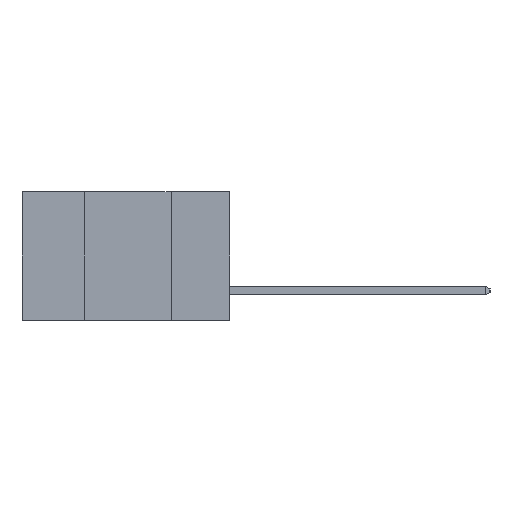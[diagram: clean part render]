
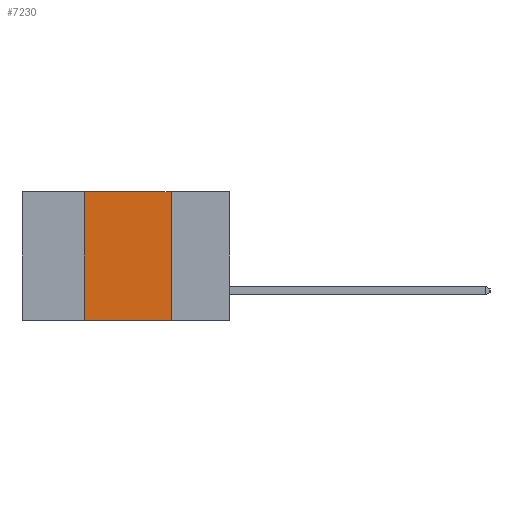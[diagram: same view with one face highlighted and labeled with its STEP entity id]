
A CAD part, left-side view. The second image highlights one B-rep face of the part: STEP entity #7230.
In plain terms, the highlighted planar face has unit normal (-1, 0, 0).
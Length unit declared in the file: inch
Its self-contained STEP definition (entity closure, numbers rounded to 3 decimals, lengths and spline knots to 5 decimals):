
#429 = VECTOR ( 'NONE', #4932, 39.37008 ) ;
#771 = AXIS2_PLACEMENT_3D ( 'NONE', #3577, #3506, #3486 ) ;
#937 = LINE ( 'NONE', #2369, #7788 ) ;
#1126 = FACE_OUTER_BOUND ( 'NONE', #3148, .T. ) ;
#1484 = VECTOR ( 'NONE', #6190, 39.37008 ) ;
#2097 = CARTESIAN_POINT ( 'NONE',  ( 0., 0.17, -0.37 ) ) ;
#2140 = EDGE_CURVE ( 'NONE', #3758, #3508, #8169, .T. ) ;
#2243 = DIRECTION ( 'NONE',  ( 0., -1., 0. ) ) ;
#2342 = LINE ( 'NONE', #4279, #429 ) ;
#2369 = CARTESIAN_POINT ( 'NONE',  ( 0., 0.6, -0.37 ) ) ;
#2577 = VERTEX_POINT ( 'NONE', #4008 ) ;
#3101 = LINE ( 'NONE', #8383, #1484 ) ;
#3103 = VECTOR ( 'NONE', #4259, 39.37008 ) ;
#3148 = EDGE_LOOP ( 'NONE', ( #3503, #3514, #3534, #3542 ) ) ;
#3486 = DIRECTION ( 'NONE',  ( 0., 0., -1. ) ) ;
#3503 = ORIENTED_EDGE ( 'NONE', *, *, #8331, .F. ) ;
#3506 = DIRECTION ( 'NONE',  ( 1., 0., 0. ) ) ;
#3508 = VERTEX_POINT ( 'NONE', #7822 ) ;
#3514 = ORIENTED_EDGE ( 'NONE', *, *, #6528, .F. ) ;
#3534 = ORIENTED_EDGE ( 'NONE', *, *, #2140, .F. ) ;
#3542 = ORIENTED_EDGE ( 'NONE', *, *, #5320, .T. ) ;
#3577 = CARTESIAN_POINT ( 'NONE',  ( 0., 0.6, 0. ) ) ;
#3758 = VERTEX_POINT ( 'NONE', #5098 ) ;
#3777 = PLANE ( 'NONE',  #771 ) ;
#4008 = CARTESIAN_POINT ( 'NONE',  ( 0., 0.17, 0. ) ) ;
#4259 = DIRECTION ( 'NONE',  ( 0., 0., 1. ) ) ;
#4279 = CARTESIAN_POINT ( 'NONE',  ( 0., 0.17, -0.37 ) ) ;
#4932 = DIRECTION ( 'NONE',  ( 0., 0., -1. ) ) ;
#5098 = CARTESIAN_POINT ( 'NONE',  ( 0., 0.42, -0.37 ) ) ;
#5320 = EDGE_CURVE ( 'NONE', #3758, #5357, #937, .T. ) ;
#5357 = VERTEX_POINT ( 'NONE', #2097 ) ;
#6190 = DIRECTION ( 'NONE',  ( 0., -1., 0. ) ) ;
#6528 = EDGE_CURVE ( 'NONE', #3508, #2577, #3101, .T. ) ;
#7230 = ADVANCED_FACE ( 'NONE', ( #1126 ), #3777, .F. ) ;
#7499 = CARTESIAN_POINT ( 'NONE',  ( 0., 0.42, -0.37 ) ) ;
#7788 = VECTOR ( 'NONE', #2243, 39.37008 ) ;
#7822 = CARTESIAN_POINT ( 'NONE',  ( 0., 0.42, 0. ) ) ;
#8169 = LINE ( 'NONE', #7499, #3103 ) ;
#8331 = EDGE_CURVE ( 'NONE', #2577, #5357, #2342, .T. ) ;
#8383 = CARTESIAN_POINT ( 'NONE',  ( 0., 0.6, 0. ) ) ;
